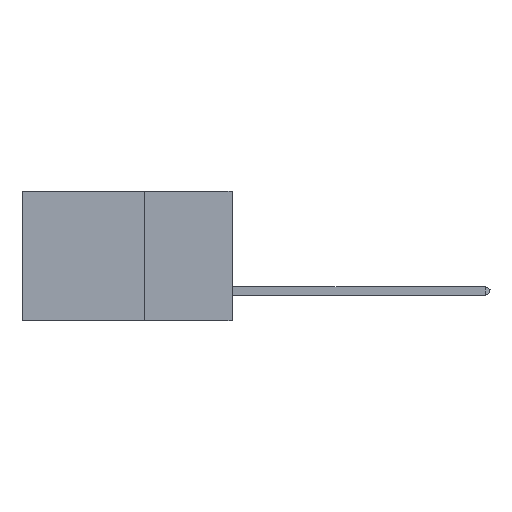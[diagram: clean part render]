
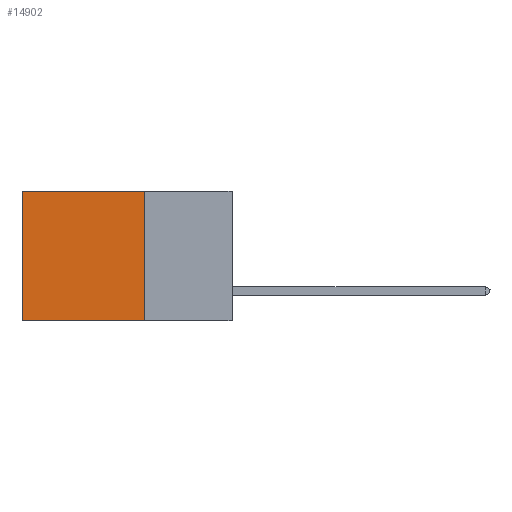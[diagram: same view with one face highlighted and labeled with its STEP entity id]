
A CAD part, left-side view. The second image highlights one B-rep face of the part: STEP entity #14902.
In plain terms, the highlighted planar face has unit normal (-1, 0, 0).
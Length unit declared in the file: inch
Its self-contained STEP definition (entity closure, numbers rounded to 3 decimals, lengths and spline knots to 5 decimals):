
#469 = ORIENTED_EDGE ( 'NONE', *, *, #41296, .T. ) ;
#880 = CARTESIAN_POINT ( 'NONE',  ( 0.2875, 0.6, -0.37 ) ) ;
#1239 = FACE_OUTER_BOUND ( 'NONE', #23231, .T. ) ;
#3083 = EDGE_CURVE ( 'NONE', #40522, #40978, #12113, .T. ) ;
#3355 = VECTOR ( 'NONE', #25169, 39.37008 ) ;
#3711 = CARTESIAN_POINT ( 'NONE',  ( 0.2875, 0.25, 0. ) ) ;
#6105 = VERTEX_POINT ( 'NONE', #9367 ) ;
#9367 = CARTESIAN_POINT ( 'NONE',  ( 0.2875, 0.6, 0. ) ) ;
#9797 = ORIENTED_EDGE ( 'NONE', *, *, #36329, .F. ) ;
#12113 = LINE ( 'NONE', #40559, #23346 ) ;
#14053 = ORIENTED_EDGE ( 'NONE', *, *, #3083, .F. ) ;
#14672 = VERTEX_POINT ( 'NONE', #29658 ) ;
#14902 = ADVANCED_FACE ( 'NONE', ( #1239 ), #22395, .F. ) ;
#16279 = DIRECTION ( 'NONE',  ( 1., 0., 0. ) ) ;
#18866 = LINE ( 'NONE', #28971, #3355 ) ;
#20338 = AXIS2_PLACEMENT_3D ( 'NONE', #29042, #16279, #39702 ) ;
#22352 = VECTOR ( 'NONE', #40786, 39.37008 ) ;
#22395 = PLANE ( 'NONE',  #20338 ) ;
#23231 = EDGE_LOOP ( 'NONE', ( #24393, #14053, #9797, #469 ) ) ;
#23346 = VECTOR ( 'NONE', #23829, 39.37008 ) ;
#23829 = DIRECTION ( 'NONE',  ( 0., 1., 0. ) ) ;
#24208 = DIRECTION ( 'NONE',  ( 0., 0., -1. ) ) ;
#24393 = ORIENTED_EDGE ( 'NONE', *, *, #28899, .T. ) ;
#25169 = DIRECTION ( 'NONE',  ( 0., 0., -1. ) ) ;
#26224 = VECTOR ( 'NONE', #24208, 39.37008 ) ;
#27837 = LINE ( 'NONE', #41360, #26224 ) ;
#28899 = EDGE_CURVE ( 'NONE', #6105, #40978, #27837, .T. ) ;
#28971 = CARTESIAN_POINT ( 'NONE',  ( 0.2875, 0.25, 0. ) ) ;
#29042 = CARTESIAN_POINT ( 'NONE',  ( 0.2875, 0.25, 0. ) ) ;
#29658 = CARTESIAN_POINT ( 'NONE',  ( 0.2875, 0.25, 0. ) ) ;
#36308 = LINE ( 'NONE', #3711, #22352 ) ;
#36329 = EDGE_CURVE ( 'NONE', #14672, #40522, #18866, .T. ) ;
#39702 = DIRECTION ( 'NONE',  ( 0., 0., -1. ) ) ;
#40522 = VERTEX_POINT ( 'NONE', #42792 ) ;
#40559 = CARTESIAN_POINT ( 'NONE',  ( 0.2875, 0.25, -0.37 ) ) ;
#40786 = DIRECTION ( 'NONE',  ( 0., 1., 0. ) ) ;
#40978 = VERTEX_POINT ( 'NONE', #880 ) ;
#41296 = EDGE_CURVE ( 'NONE', #14672, #6105, #36308, .T. ) ;
#41360 = CARTESIAN_POINT ( 'NONE',  ( 0.2875, 0.6, 0. ) ) ;
#42792 = CARTESIAN_POINT ( 'NONE',  ( 0.2875, 0.25, -0.37 ) ) ;
